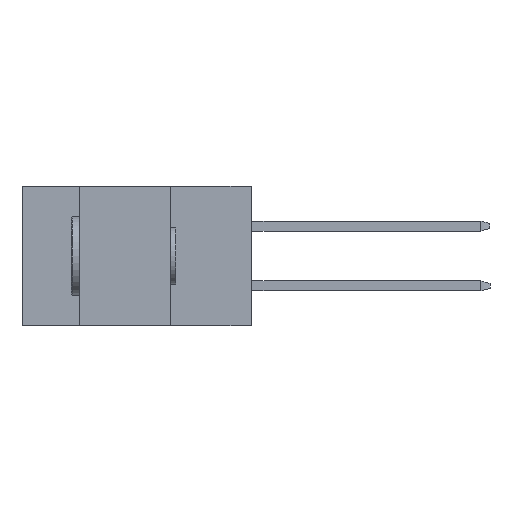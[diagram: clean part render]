
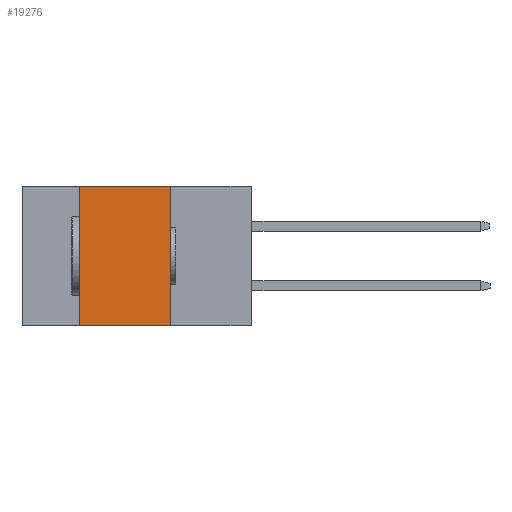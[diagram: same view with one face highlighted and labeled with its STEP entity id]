
A CAD part, left-side view. The second image highlights one B-rep face of the part: STEP entity #19276.
In plain terms, the highlighted planar face has unit normal (-1, 0, 0).
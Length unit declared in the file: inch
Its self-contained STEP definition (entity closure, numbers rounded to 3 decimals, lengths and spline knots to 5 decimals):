
#7 = EDGE_CURVE ( 'NONE', #7802, #11601, #15548, .T. ) ;
#318 = ORIENTED_EDGE ( 'NONE', *, *, #9223, .T. ) ;
#556 = ORIENTED_EDGE ( 'NONE', *, *, #10641, .F. ) ;
#894 = EDGE_LOOP ( 'NONE', ( #556, #2890, #11645, #318 ) ) ;
#1056 = VECTOR ( 'NONE', #16148, 39.37008 ) ;
#1136 = EDGE_CURVE ( 'NONE', #11601, #18113, #12665, .T. ) ;
#2890 = ORIENTED_EDGE ( 'NONE', *, *, #1136, .F. ) ;
#3523 = VECTOR ( 'NONE', #18810, 39.37008 ) ;
#4120 = CARTESIAN_POINT ( 'NONE',  ( 0., 0.54, -0.437 ) ) ;
#4820 = CARTESIAN_POINT ( 'NONE',  ( 0., 0.72, 0. ) ) ;
#5870 = VECTOR ( 'NONE', #16376, 39.37008 ) ;
#7802 = VERTEX_POINT ( 'NONE', #16496 ) ;
#8057 = PLANE ( 'NONE',  #9382 ) ;
#9223 = EDGE_CURVE ( 'NONE', #7802, #11780, #12635, .T. ) ;
#9382 = AXIS2_PLACEMENT_3D ( 'NONE', #4820, #20216, #20109 ) ;
#9936 = CARTESIAN_POINT ( 'NONE',  ( 0., 0.254, -0.437 ) ) ;
#10620 = CARTESIAN_POINT ( 'NONE',  ( 0., 0.254, 0. ) ) ;
#10641 = EDGE_CURVE ( 'NONE', #18113, #11780, #16501, .T. ) ;
#11253 = VECTOR ( 'NONE', #14267, 39.37008 ) ;
#11601 = VERTEX_POINT ( 'NONE', #18723 ) ;
#11645 = ORIENTED_EDGE ( 'NONE', *, *, #7, .F. ) ;
#11780 = VERTEX_POINT ( 'NONE', #16751 ) ;
#12635 = LINE ( 'NONE', #12847, #11253 ) ;
#12665 = LINE ( 'NONE', #14417, #1056 ) ;
#12847 = CARTESIAN_POINT ( 'NONE',  ( 0., 0.72, -0.437 ) ) ;
#14267 = DIRECTION ( 'NONE',  ( 0., -1., 0. ) ) ;
#14417 = CARTESIAN_POINT ( 'NONE',  ( 0., 0.72, 0. ) ) ;
#15548 = LINE ( 'NONE', #4120, #3523 ) ;
#16148 = DIRECTION ( 'NONE',  ( 0., -1., 0. ) ) ;
#16363 = FACE_OUTER_BOUND ( 'NONE', #894, .T. ) ;
#16376 = DIRECTION ( 'NONE',  ( 0., 0., -1. ) ) ;
#16496 = CARTESIAN_POINT ( 'NONE',  ( 0., 0.54, -0.437 ) ) ;
#16501 = LINE ( 'NONE', #9936, #5870 ) ;
#16751 = CARTESIAN_POINT ( 'NONE',  ( 0., 0.254, -0.437 ) ) ;
#18113 = VERTEX_POINT ( 'NONE', #10620 ) ;
#18723 = CARTESIAN_POINT ( 'NONE',  ( 0., 0.54, 0. ) ) ;
#18810 = DIRECTION ( 'NONE',  ( 0., 0., 1. ) ) ;
#19276 = ADVANCED_FACE ( 'NONE', ( #16363 ), #8057, .F. ) ;
#20109 = DIRECTION ( 'NONE',  ( 0., 0., -1. ) ) ;
#20216 = DIRECTION ( 'NONE',  ( 1., 0., 0. ) ) ;
